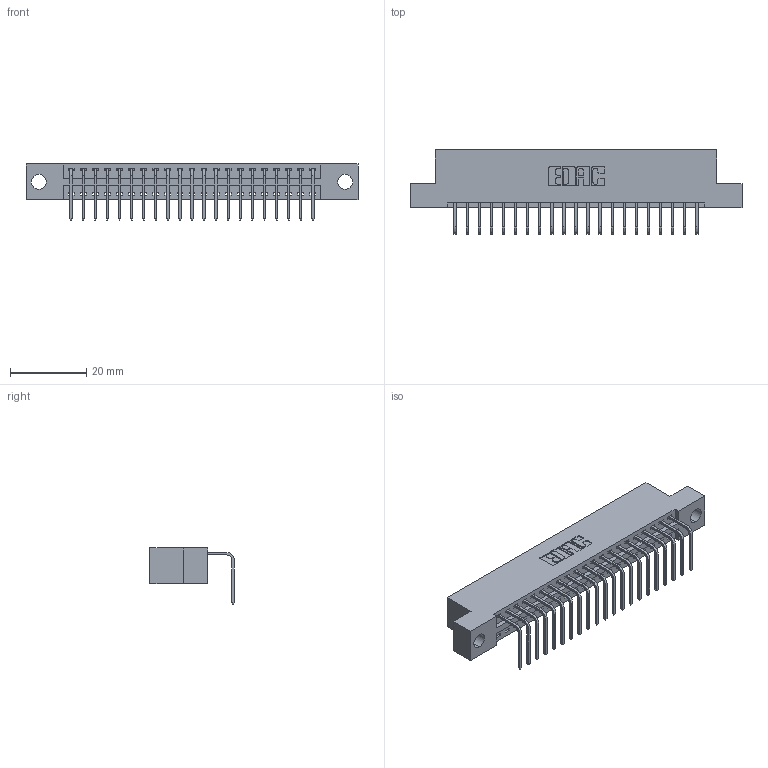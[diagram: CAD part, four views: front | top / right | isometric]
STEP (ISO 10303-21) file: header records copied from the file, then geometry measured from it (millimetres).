
FILE_DESCRIPTION (( 'STEP AP203' ), '1' );
FILE_NAME ('346-021-558-104.STEP', '2022-05-05T18:32:09', ( '' ), ( '' ), 'SwSTEP 2.0', 'SolidWorks 2020', '' );
FILE_SCHEMA (( 'CONFIG_CONTROL_DESIGN' ));
Length unit declared in the file: inch
Products named in the file (3): 346-021-558-104; 346 Part_Flush Mounting Lugs - 0.156 Dia-TH; 345-292-001_558 Tail - 2
Assembly tree (22 placements, depth 2):
  346-021-558-104
    346 Part_Flush Mounting Lugs - 0.156 Dia-TH
    345-292-001_558 Tail - 2  x21
Bounding box: 87.25 x 22.16 x 14.73 mm (x, y, z)
Volume: 8171 mm3; surface area: 10240.7 mm2
Topology: 22 solids, 22 shells, 1396 faces, 4187 edges, 2762 vertices
Faces by surface type: plane 972, cylinder 424
Entity records: 16363 total; most frequent: CARTESIAN_POINT 2821, ORIENTED_EDGE 2774, DIRECTION 2513, EDGE_CURVE 1387, VECTOR 1171, LINE 1171, VERTEX_POINT 922, AXIS2_PLACEMENT_3D 671
